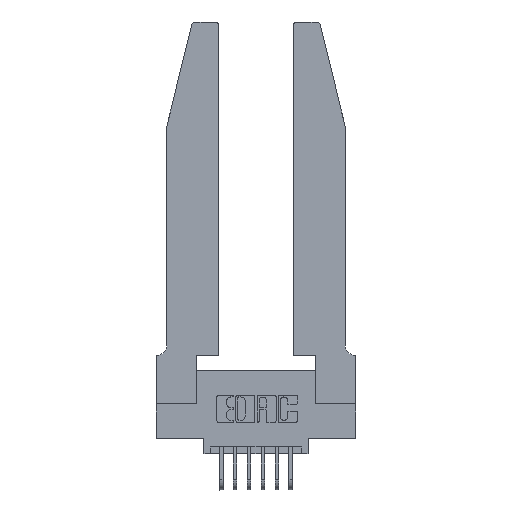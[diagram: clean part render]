
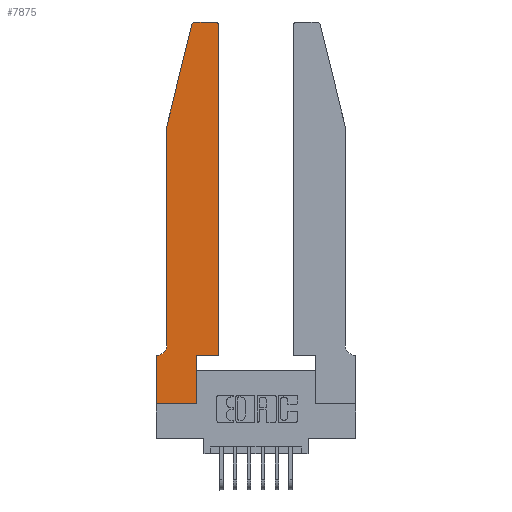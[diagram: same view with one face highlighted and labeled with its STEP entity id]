
A CAD part, top view. The second image highlights one B-rep face of the part: STEP entity #7875.
In plain terms, the highlighted planar face has unit normal (0, 0, 1).
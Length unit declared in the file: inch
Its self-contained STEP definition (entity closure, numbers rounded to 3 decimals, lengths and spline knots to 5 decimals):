
#44 = CARTESIAN_POINT ( 'NONE',  ( 0.284, 2.72, 0.37 ) ) ;
#75 = VECTOR ( 'NONE', #10194, 39.37008 ) ;
#88 = ORIENTED_EDGE ( 'NONE', *, *, #8936, .T. ) ;
#150 = CARTESIAN_POINT ( 'NONE',  ( 0., 0., 0.37 ) ) ;
#312 = LINE ( 'NONE', #150, #75 ) ;
#392 = ORIENTED_EDGE ( 'NONE', *, *, #2544, .T. ) ;
#523 = ORIENTED_EDGE ( 'NONE', *, *, #10145, .T. ) ;
#551 = AXIS2_PLACEMENT_3D ( 'NONE', #12027, #5738, #12891 ) ;
#627 = ORIENTED_EDGE ( 'NONE', *, *, #8000, .T. ) ;
#650 = EDGE_CURVE ( 'NONE', #13424, #4962, #3442, .T. ) ;
#1043 = EDGE_CURVE ( 'NONE', #4962, #3539, #1203, .T. ) ;
#1155 = VECTOR ( 'NONE', #10016, 39.37008 ) ;
#1203 = LINE ( 'NONE', #7193, #1155 ) ;
#1368 = ORIENTED_EDGE ( 'NONE', *, *, #2549, .T. ) ;
#1382 = EDGE_CURVE ( 'NONE', #3539, #8092, #5631, .T. ) ;
#1406 = EDGE_CURVE ( 'NONE', #9774, #13424, #8371, .T. ) ;
#1518 = CARTESIAN_POINT ( 'NONE',  ( 0.4505, 0.35, 0.37 ) ) ;
#1569 = DIRECTION ( 'NONE',  ( 1., 0., 0. ) ) ;
#1586 = ORIENTED_EDGE ( 'NONE', *, *, #1678, .T. ) ;
#1599 = CARTESIAN_POINT ( 'NONE',  ( 0.25487, 2.72718, 0.37 ) ) ;
#1678 = EDGE_CURVE ( 'NONE', #2227, #4452, #3011, .T. ) ;
#1741 = ORIENTED_EDGE ( 'NONE', *, *, #13000, .T. ) ;
#1998 = CARTESIAN_POINT ( 'NONE',  ( 0.0755, 2., 0.37 ) ) ;
#2211 = ORIENTED_EDGE ( 'NONE', *, *, #1406, .T. ) ;
#2223 = DIRECTION ( 'NONE',  ( 0., 0., 1. ) ) ;
#2227 = VERTEX_POINT ( 'NONE', #12108 ) ;
#2275 = ORIENTED_EDGE ( 'NONE', *, *, #650, .T. ) ;
#2544 = EDGE_CURVE ( 'NONE', #2776, #14119, #7651, .T. ) ;
#2549 = EDGE_CURVE ( 'NONE', #8046, #2227, #7544, .T. ) ;
#2573 = EDGE_CURVE ( 'NONE', #8092, #12423, #7364, .T. ) ;
#2706 = ORIENTED_EDGE ( 'NONE', *, *, #1043, .T. ) ;
#2776 = VERTEX_POINT ( 'NONE', #12692 ) ;
#2840 = VECTOR ( 'NONE', #13954, 39.37008 ) ;
#3011 = LINE ( 'NONE', #11103, #3963 ) ;
#3079 = ORIENTED_EDGE ( 'NONE', *, *, #1382, .T. ) ;
#3251 = CARTESIAN_POINT ( 'NONE',  ( 0., 0.35, 0.37 ) ) ;
#3369 = ORIENTED_EDGE ( 'NONE', *, *, #2573, .T. ) ;
#3393 = VECTOR ( 'NONE', #7938, 39.37008 ) ;
#3442 = LINE ( 'NONE', #7689, #3393 ) ;
#3539 = VERTEX_POINT ( 'NONE', #1518 ) ;
#3639 = DIRECTION ( 'NONE',  ( -0.239, -0.971, 0. ) ) ;
#3963 = VECTOR ( 'NONE', #4450, 39.37008 ) ;
#4007 = CARTESIAN_POINT ( 'NONE',  ( 0.2865, 0.35, 0.37 ) ) ;
#4450 = DIRECTION ( 'NONE',  ( -1., 0., 0. ) ) ;
#4452 = VERTEX_POINT ( 'NONE', #13743 ) ;
#4501 = VECTOR ( 'NONE', #12229, 39.37008 ) ;
#4520 = LINE ( 'NONE', #1998, #4501 ) ;
#4621 = DIRECTION ( 'NONE',  ( 1., 0., 0. ) ) ;
#4933 = CARTESIAN_POINT ( 'NONE',  ( 0.0755, 0.42, 0.37 ) ) ;
#4962 = VERTEX_POINT ( 'NONE', #4007 ) ;
#5017 = DIRECTION ( 'NONE',  ( -1., 0., 0. ) ) ;
#5215 = VECTOR ( 'NONE', #12272, 39.37008 ) ;
#5631 = LINE ( 'NONE', #13898, #5215 ) ;
#5738 = DIRECTION ( 'NONE',  ( 0., 0., -1. ) ) ;
#6548 = LINE ( 'NONE', #10353, #7137 ) ;
#6634 = FACE_OUTER_BOUND ( 'NONE', #9965, .T. ) ;
#7137 = VECTOR ( 'NONE', #5017, 39.37008 ) ;
#7193 = CARTESIAN_POINT ( 'NONE',  ( 0.4505, 0.35, 0.37 ) ) ;
#7364 = CIRCLE ( 'NONE', #11609, 0.03 ) ;
#7544 = CIRCLE ( 'NONE', #551, 0.07 ) ;
#7651 = CIRCLE ( 'NONE', #12819, 0.03 ) ;
#7689 = CARTESIAN_POINT ( 'NONE',  ( 0.2865, 0.35, 0.37 ) ) ;
#7875 = ADVANCED_FACE ( 'NONE', ( #6634 ), #9274, .T. ) ;
#7938 = DIRECTION ( 'NONE',  ( 0., 1., 0. ) ) ;
#8000 = EDGE_CURVE ( 'NONE', #8433, #8046, #4520, .T. ) ;
#8046 = VERTEX_POINT ( 'NONE', #4933 ) ;
#8092 = VERTEX_POINT ( 'NONE', #9541 ) ;
#8371 = LINE ( 'NONE', #8453, #2840 ) ;
#8433 = VERTEX_POINT ( 'NONE', #9954 ) ;
#8453 = CARTESIAN_POINT ( 'NONE',  ( 0., 0., 0.37 ) ) ;
#8479 = CARTESIAN_POINT ( 'NONE',  ( 0.2865, 0., 0.37 ) ) ;
#8936 = EDGE_CURVE ( 'NONE', #12423, #2776, #6548, .T. ) ;
#9092 = DIRECTION ( 'NONE',  ( 0., 0., 1. ) ) ;
#9274 = PLANE ( 'NONE',  #11572 ) ;
#9514 = CARTESIAN_POINT ( 'NONE',  ( 0.4205, 2.72, 0.37 ) ) ;
#9541 = CARTESIAN_POINT ( 'NONE',  ( 0.4505, 2.72, 0.37 ) ) ;
#9774 = VERTEX_POINT ( 'NONE', #13900 ) ;
#9954 = CARTESIAN_POINT ( 'NONE',  ( 0.0755, 2., 0.37 ) ) ;
#9965 = EDGE_LOOP ( 'NONE', ( #88, #392, #523, #627, #1368, #1586, #1741, #2211, #2275, #2706, #3079, #3369 ) ) ;
#10016 = DIRECTION ( 'NONE',  ( 1., 0., 0. ) ) ;
#10145 = EDGE_CURVE ( 'NONE', #14119, #8433, #10960, .T. ) ;
#10194 = DIRECTION ( 'NONE',  ( 0., -1., 0. ) ) ;
#10223 = VECTOR ( 'NONE', #3639, 39.37008 ) ;
#10353 = CARTESIAN_POINT ( 'NONE',  ( 0.2605, 2.75, 0.37 ) ) ;
#10553 = DIRECTION ( 'NONE',  ( 1., 0., 0. ) ) ;
#10576 = CARTESIAN_POINT ( 'NONE',  ( 0.0755, 2., 0.37 ) ) ;
#10960 = LINE ( 'NONE', #10576, #10223 ) ;
#11103 = CARTESIAN_POINT ( 'NONE',  ( 0.0755, 0.35, 0.37 ) ) ;
#11241 = DIRECTION ( 'NONE',  ( 0., 0., 1. ) ) ;
#11572 = AXIS2_PLACEMENT_3D ( 'NONE', #3251, #11241, #4621 ) ;
#11609 = AXIS2_PLACEMENT_3D ( 'NONE', #9514, #2223, #10553 ) ;
#12027 = CARTESIAN_POINT ( 'NONE',  ( 0.0055, 0.42, 0.37 ) ) ;
#12108 = CARTESIAN_POINT ( 'NONE',  ( 0.0055, 0.35, 0.37 ) ) ;
#12229 = DIRECTION ( 'NONE',  ( 0., -1., 0. ) ) ;
#12272 = DIRECTION ( 'NONE',  ( 0., 1., 0. ) ) ;
#12423 = VERTEX_POINT ( 'NONE', #13395 ) ;
#12692 = CARTESIAN_POINT ( 'NONE',  ( 0.284, 2.75, 0.37 ) ) ;
#12819 = AXIS2_PLACEMENT_3D ( 'NONE', #44, #9092, #1569 ) ;
#12891 = DIRECTION ( 'NONE',  ( -1., 0., 0. ) ) ;
#13000 = EDGE_CURVE ( 'NONE', #4452, #9774, #312, .T. ) ;
#13395 = CARTESIAN_POINT ( 'NONE',  ( 0.4205, 2.75, 0.37 ) ) ;
#13424 = VERTEX_POINT ( 'NONE', #8479 ) ;
#13743 = CARTESIAN_POINT ( 'NONE',  ( 0., 0.35, 0.37 ) ) ;
#13898 = CARTESIAN_POINT ( 'NONE',  ( 0.4505, 0.35, 0.37 ) ) ;
#13900 = CARTESIAN_POINT ( 'NONE',  ( 0., 0., 0.37 ) ) ;
#13954 = DIRECTION ( 'NONE',  ( 1., 0., 0. ) ) ;
#14119 = VERTEX_POINT ( 'NONE', #1599 ) ;
